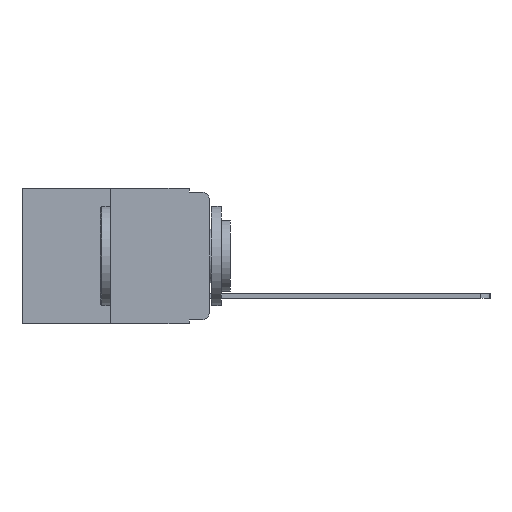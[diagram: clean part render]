
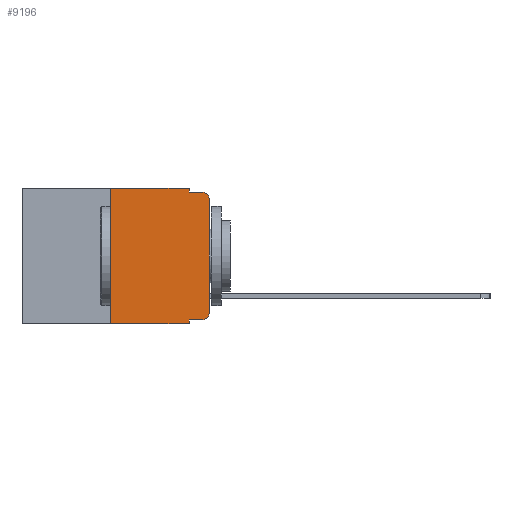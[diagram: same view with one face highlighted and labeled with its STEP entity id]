
A CAD part, left-side view. The second image highlights one B-rep face of the part: STEP entity #9196.
In plain terms, the highlighted planar face has unit normal (-1, 0, 0).
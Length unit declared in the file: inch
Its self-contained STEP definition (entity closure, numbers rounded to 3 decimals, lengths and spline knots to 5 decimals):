
#7 = ORIENTED_EDGE ( 'NONE', *, *, #4044, .T. ) ;
#99 = CARTESIAN_POINT ( 'NONE',  ( 0., 0.051, -0.333 ) ) ;
#353 = ORIENTED_EDGE ( 'NONE', *, *, #2815, .F. ) ;
#486 = VERTEX_POINT ( 'NONE', #7308 ) ;
#504 = DIRECTION ( 'NONE',  ( 0., 0., -1. ) ) ;
#519 = DIRECTION ( 'NONE',  ( -1., 0., 0. ) ) ;
#547 = CARTESIAN_POINT ( 'NONE',  ( 0., 0.02, -0.313 ) ) ;
#640 = CARTESIAN_POINT ( 'NONE',  ( 0., 0., 0. ) ) ;
#861 = VECTOR ( 'NONE', #2908, 39.37008 ) ;
#1005 = ORIENTED_EDGE ( 'NONE', *, *, #1976, .F. ) ;
#1040 = AXIS2_PLACEMENT_3D ( 'NONE', #1792, #5933, #5873 ) ;
#1219 = VECTOR ( 'NONE', #1610, 39.37008 ) ;
#1610 = DIRECTION ( 'NONE',  ( 0., -1., 0. ) ) ;
#1774 = FACE_OUTER_BOUND ( 'NONE', #6172, .T. ) ;
#1792 = CARTESIAN_POINT ( 'NONE',  ( 0., 0.02, -0.03 ) ) ;
#1862 = CARTESIAN_POINT ( 'NONE',  ( 0., 0.051, 0. ) ) ;
#1976 = EDGE_CURVE ( 'NONE', #5019, #9656, #3735, .T. ) ;
#2109 = CARTESIAN_POINT ( 'NONE',  ( 0., 0.473, 0. ) ) ;
#2234 = LINE ( 'NONE', #99, #7116 ) ;
#2235 = CARTESIAN_POINT ( 'NONE',  ( 0., 0.051, -0.01 ) ) ;
#2333 = ORIENTED_EDGE ( 'NONE', *, *, #7393, .T. ) ;
#2424 = EDGE_CURVE ( 'NONE', #3864, #6355, #2234, .T. ) ;
#2815 = EDGE_CURVE ( 'NONE', #4091, #6397, #8821, .T. ) ;
#2843 = DIRECTION ( 'NONE',  ( 0., -1., 0. ) ) ;
#2908 = DIRECTION ( 'NONE',  ( 0., 0., -1. ) ) ;
#3456 = CARTESIAN_POINT ( 'NONE',  ( 0., 0.051, -0.343 ) ) ;
#3527 = VECTOR ( 'NONE', #7040, 39.37008 ) ;
#3628 = DIRECTION ( 'NONE',  ( 0., 0., 1. ) ) ;
#3679 = EDGE_CURVE ( 'NONE', #3864, #6772, #3687, .T. ) ;
#3687 = LINE ( 'NONE', #1862, #861 ) ;
#3735 = LINE ( 'NONE', #2109, #1219 ) ;
#3864 = VERTEX_POINT ( 'NONE', #6737 ) ;
#4044 = EDGE_CURVE ( 'NONE', #486, #6397, #10761, .T. ) ;
#4070 = ORIENTED_EDGE ( 'NONE', *, *, #10746, .T. ) ;
#4091 = VERTEX_POINT ( 'NONE', #2235 ) ;
#4185 = CARTESIAN_POINT ( 'NONE',  ( 0., 0.25, 0. ) ) ;
#4256 = LINE ( 'NONE', #4185, #10541 ) ;
#4269 = CARTESIAN_POINT ( 'NONE',  ( 0., 0.02, -0.01 ) ) ;
#4396 = VECTOR ( 'NONE', #7400, 39.37008 ) ;
#4474 = DIRECTION ( 'NONE',  ( 0., 0., 1. ) ) ;
#5019 = VERTEX_POINT ( 'NONE', #6583 ) ;
#5204 = CARTESIAN_POINT ( 'NONE',  ( 0., 0.051, 0. ) ) ;
#5367 = PLANE ( 'NONE',  #8671 ) ;
#5399 = CARTESIAN_POINT ( 'NONE',  ( 0., 0.473, -0.343 ) ) ;
#5525 = CARTESIAN_POINT ( 'NONE',  ( 0., 0.02, -0.333 ) ) ;
#5553 = ORIENTED_EDGE ( 'NONE', *, *, #9800, .F. ) ;
#5595 = VECTOR ( 'NONE', #3628, 39.37008 ) ;
#5678 = VECTOR ( 'NONE', #6211, 39.37008 ) ;
#5873 = DIRECTION ( 'NONE',  ( 0., 0., -1. ) ) ;
#5933 = DIRECTION ( 'NONE',  ( -1., 0., 0. ) ) ;
#6055 = ORIENTED_EDGE ( 'NONE', *, *, #7607, .F. ) ;
#6144 = CARTESIAN_POINT ( 'NONE',  ( 0., 0.473, 0. ) ) ;
#6171 = DIRECTION ( 'NONE',  ( 0., 0., -1. ) ) ;
#6172 = EDGE_LOOP ( 'NONE', ( #2333, #7, #353, #5553, #1005, #6055, #4070, #10864, #7063, #7323 ) ) ;
#6211 = DIRECTION ( 'NONE',  ( 0., -1., 0. ) ) ;
#6223 = AXIS2_PLACEMENT_3D ( 'NONE', #547, #519, #504 ) ;
#6232 = CARTESIAN_POINT ( 'NONE',  ( 0., 0.051, 0. ) ) ;
#6355 = VERTEX_POINT ( 'NONE', #5525 ) ;
#6397 = VERTEX_POINT ( 'NONE', #4269 ) ;
#6583 = CARTESIAN_POINT ( 'NONE',  ( 0., 0.25, 0. ) ) ;
#6693 = EDGE_CURVE ( 'NONE', #6355, #7583, #11166, .T. ) ;
#6737 = CARTESIAN_POINT ( 'NONE',  ( 0., 0.051, -0.333 ) ) ;
#6772 = VERTEX_POINT ( 'NONE', #3456 ) ;
#7040 = DIRECTION ( 'NONE',  ( 0., 0., -1. ) ) ;
#7063 = ORIENTED_EDGE ( 'NONE', *, *, #2424, .T. ) ;
#7116 = VECTOR ( 'NONE', #2843, 39.37008 ) ;
#7158 = CARTESIAN_POINT ( 'NONE',  ( 0., 0.051, -0.01 ) ) ;
#7308 = CARTESIAN_POINT ( 'NONE',  ( 0., 0., -0.03 ) ) ;
#7323 = ORIENTED_EDGE ( 'NONE', *, *, #6693, .T. ) ;
#7393 = EDGE_CURVE ( 'NONE', #7583, #486, #7776, .T. ) ;
#7400 = DIRECTION ( 'NONE',  ( 0., -1., 0. ) ) ;
#7583 = VERTEX_POINT ( 'NONE', #7968 ) ;
#7607 = EDGE_CURVE ( 'NONE', #10465, #5019, #4256, .T. ) ;
#7776 = LINE ( 'NONE', #640, #5595 ) ;
#7968 = CARTESIAN_POINT ( 'NONE',  ( 0., 0., -0.313 ) ) ;
#8671 = AXIS2_PLACEMENT_3D ( 'NONE', #6144, #11022, #6171 ) ;
#8821 = LINE ( 'NONE', #7158, #4396 ) ;
#9196 = ADVANCED_FACE ( 'NONE', ( #1774 ), #5367, .F. ) ;
#9656 = VERTEX_POINT ( 'NONE', #5204 ) ;
#9799 = CARTESIAN_POINT ( 'NONE',  ( 0., 0.25, -0.343 ) ) ;
#9800 = EDGE_CURVE ( 'NONE', #9656, #4091, #10136, .T. ) ;
#9997 = LINE ( 'NONE', #5399, #5678 ) ;
#10136 = LINE ( 'NONE', #6232, #3527 ) ;
#10465 = VERTEX_POINT ( 'NONE', #9799 ) ;
#10541 = VECTOR ( 'NONE', #4474, 39.37008 ) ;
#10746 = EDGE_CURVE ( 'NONE', #10465, #6772, #9997, .T. ) ;
#10761 = CIRCLE ( 'NONE', #1040, 0.02 ) ;
#10864 = ORIENTED_EDGE ( 'NONE', *, *, #3679, .F. ) ;
#11022 = DIRECTION ( 'NONE',  ( 1., 0., 0. ) ) ;
#11166 = CIRCLE ( 'NONE', #6223, 0.02 ) ;
